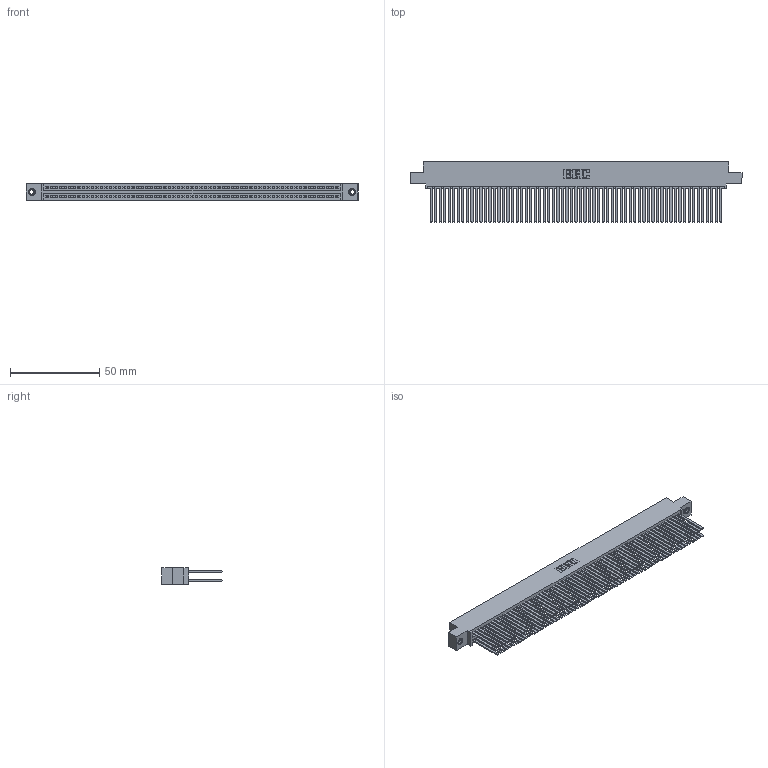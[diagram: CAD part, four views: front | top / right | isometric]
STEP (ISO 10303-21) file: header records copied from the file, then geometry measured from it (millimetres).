
FILE_DESCRIPTION (( 'STEP AP203' ), '1' );
FILE_NAME ('345-130-544-507.STEP', '2019-11-07T15:05:15', ( '' ), ( '' ), 'SwSTEP 2.0', 'SolidWorks 2016', '' );
FILE_SCHEMA (( 'CONFIG_CONTROL_DESIGN' ));
Length unit declared in the file: inch
Products named in the file (4): 345 Part_0.110 Offset - 0.156 Dia-TI; 345-250-001_345-250-005-103; 345-292-001_345-293-144; 345-130-544-507
Assembly tree (133 placements, depth 2):
  345-130-544-507
    345 Part_0.110 Offset - 0.156 Dia-TI
    345-292-001_345-293-144  x130
    345-250-001_345-250-005-103  x2
Bounding box: 186.31 x 33.96 x 9.4 mm (x, y, z)
Volume: 20047.2 mm3; surface area: 35540.5 mm2
Topology: 133 solids, 133 shells, 5910 faces, 17519 edges, 11498 vertices
Faces by surface type: plane 3886, cylinder 2008, cone 12, torus 4
Entity records: 49038 total; most frequent: CARTESIAN_POINT 8179, ORIENTED_EDGE 8106, DIRECTION 7207, EDGE_CURVE 4053, LINE 3645, VECTOR 3645, VERTEX_POINT 2696, AXIS2_PLACEMENT_3D 1781
